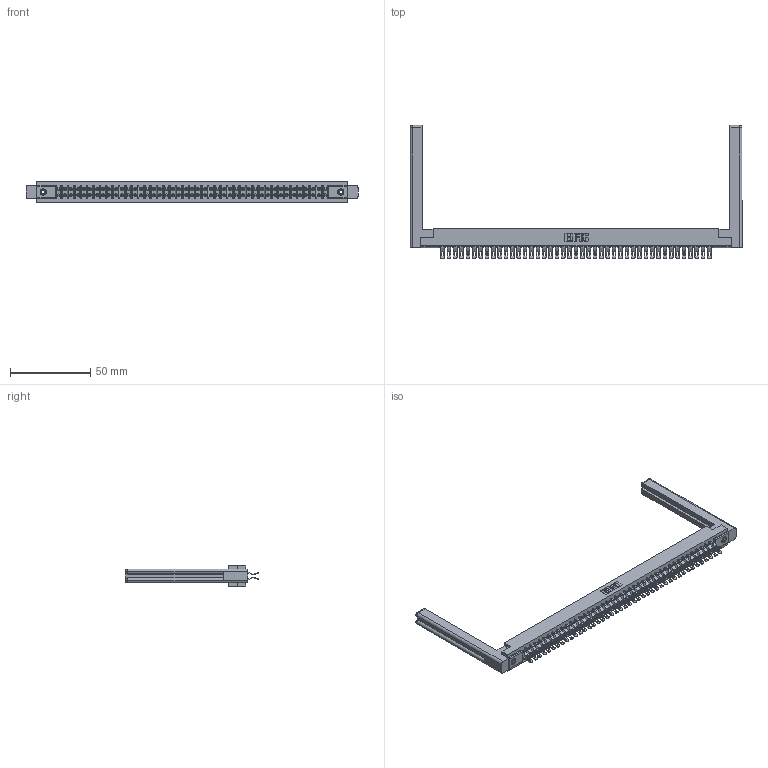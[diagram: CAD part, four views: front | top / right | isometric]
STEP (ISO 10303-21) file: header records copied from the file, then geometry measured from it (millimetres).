
FILE_DESCRIPTION (( 'STEP AP203' ), '1' );
FILE_NAME ('357-086-455-258.STEP', '2020-10-04T06:05:34', ( '' ), ( '' ), 'SwSTEP 2.0', 'SolidWorks 2020', '' );
FILE_SCHEMA (( 'CONFIG_CONTROL_DESIGN' ));
Length unit declared in the file: inch
Products named in the file (5): 307 Part_.156 Dia Mounting Holes; 307-220-058; 307-290-001_555; 345-250-001_345-250-001-102; 357-086-455-258
Assembly tree (91 placements, depth 2):
  357-086-455-258
    307 Part_.156 Dia Mounting Holes
    307-290-001_555  x86
    307-220-058  x2
    345-250-001_345-250-001-102  x2
Bounding box: 207.01 x 83.06 x 12.7 mm (x, y, z)
Volume: 29405.8 mm3; surface area: 33592.2 mm2
Topology: 91 solids, 91 shells, 5550 faces, 16243 edges, 10582 vertices
Faces by surface type: plane 3078, cylinder 2360, sphere 88, torus 12, cone 12
Entity records: 41286 total; most frequent: CARTESIAN_POINT 6778, ORIENTED_EDGE 6662, DIRECTION 6603, EDGE_CURVE 3331, LINE 2541, VECTOR 2541, VERTEX_POINT 2152, AXIS2_PLACEMENT_3D 2031
